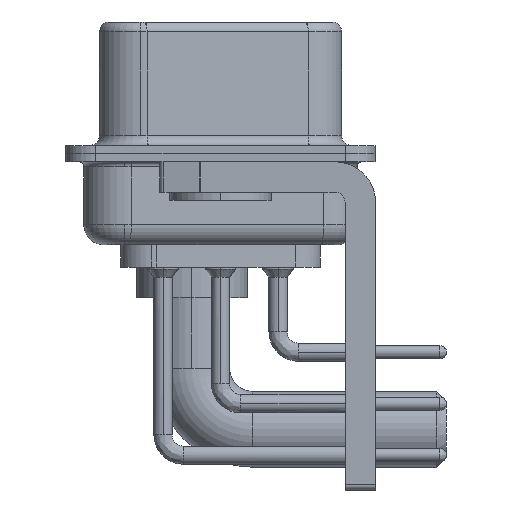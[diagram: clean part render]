
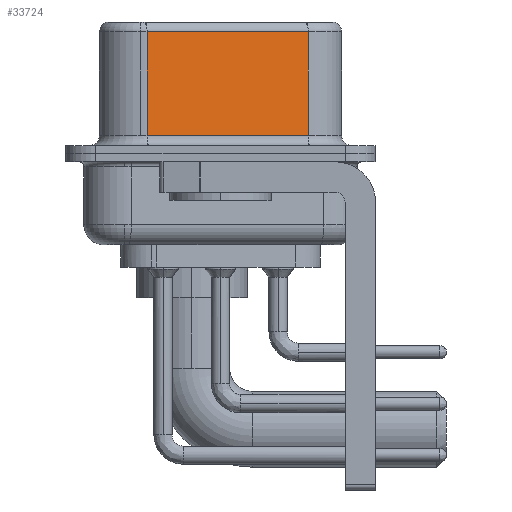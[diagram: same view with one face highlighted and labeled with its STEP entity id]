
A CAD part, left-side view. The second image highlights one B-rep face of the part: STEP entity #33724.
In plain terms, the highlighted planar face has unit normal (-0.985, -0.174, 0).
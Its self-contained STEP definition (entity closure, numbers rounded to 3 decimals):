
#979 = VERTEX_POINT ( 'NONE', #6886 ) ;
#1626 = CARTESIAN_POINT ( 'NONE',  ( 3.73, 3.628, 0.9 ) ) ;
#1787 = CARTESIAN_POINT ( 'NONE',  ( 3.73, 3.628, 6.52 ) ) ;
#2926 = CARTESIAN_POINT ( 'NONE',  ( 5.132, -4.322, 6.52 ) ) ;
#3146 = EDGE_CURVE ( 'NONE', #979, #28283, #9934, .T. ) ;
#5277 = DIRECTION ( 'NONE',  ( 0.174, -0.985, 0. ) ) ;
#5971 = EDGE_LOOP ( 'NONE', ( #12110, #14883, #33726, #27678 ) ) ;
#6455 = EDGE_CURVE ( 'NONE', #16777, #28283, #16859, .T. ) ;
#6886 = CARTESIAN_POINT ( 'NONE',  ( 5.132, -4.322, 6.02 ) ) ;
#8303 = CARTESIAN_POINT ( 'NONE',  ( 5.132, -4.322, 6.02 ) ) ;
#9218 = VERTEX_POINT ( 'NONE', #27528 ) ;
#9934 = LINE ( 'NONE', #12641, #17440 ) ;
#10797 = EDGE_CURVE ( 'NONE', #979, #9218, #34358, .T. ) ;
#11954 = DIRECTION ( 'NONE',  ( -0.174, 0.985, 0. ) ) ;
#12110 = ORIENTED_EDGE ( 'NONE', *, *, #3146, .F. ) ;
#12641 = CARTESIAN_POINT ( 'NONE',  ( 5.132, -4.322, 6.52 ) ) ;
#14668 = DIRECTION ( 'NONE',  ( 0.985, 0.174, 0. ) ) ;
#14850 = FACE_OUTER_BOUND ( 'NONE', #5971, .T. ) ;
#14883 = ORIENTED_EDGE ( 'NONE', *, *, #10797, .T. ) ;
#15265 = VECTOR ( 'NONE', #5277, 1000. ) ;
#16777 = VERTEX_POINT ( 'NONE', #1626 ) ;
#16859 = LINE ( 'NONE', #25682, #15265 ) ;
#17440 = VECTOR ( 'NONE', #36203, 1000. ) ;
#19414 = EDGE_CURVE ( 'NONE', #9218, #16777, #28369, .T. ) ;
#23127 = DIRECTION ( 'NONE',  ( 0., 0., -1. ) ) ;
#23506 = VECTOR ( 'NONE', #37668, 1000. ) ;
#25682 = CARTESIAN_POINT ( 'NONE',  ( 5.132, -4.322, 0.9 ) ) ;
#27528 = CARTESIAN_POINT ( 'NONE',  ( 3.73, 3.628, 6.02 ) ) ;
#27678 = ORIENTED_EDGE ( 'NONE', *, *, #6455, .T. ) ;
#28283 = VERTEX_POINT ( 'NONE', #30308 ) ;
#28369 = LINE ( 'NONE', #1787, #33273 ) ;
#30308 = CARTESIAN_POINT ( 'NONE',  ( 5.132, -4.322, 0.9 ) ) ;
#32628 = PLANE ( 'NONE',  #37367 ) ;
#33273 = VECTOR ( 'NONE', #23127, 1000. ) ;
#33724 = ADVANCED_FACE ( 'NONE', ( #14850 ), #32628, .F. ) ;
#33726 = ORIENTED_EDGE ( 'NONE', *, *, #19414, .T. ) ;
#34358 = LINE ( 'NONE', #8303, #23506 ) ;
#36203 = DIRECTION ( 'NONE',  ( 0., 0., -1. ) ) ;
#37367 = AXIS2_PLACEMENT_3D ( 'NONE', #2926, #14668, #11954 ) ;
#37668 = DIRECTION ( 'NONE',  ( -0.174, 0.985, 0. ) ) ;
